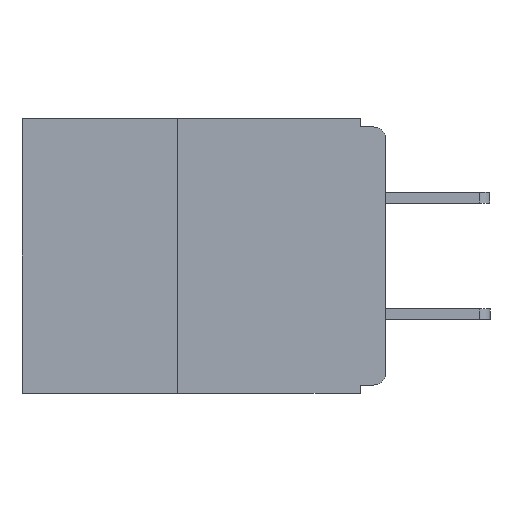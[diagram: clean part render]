
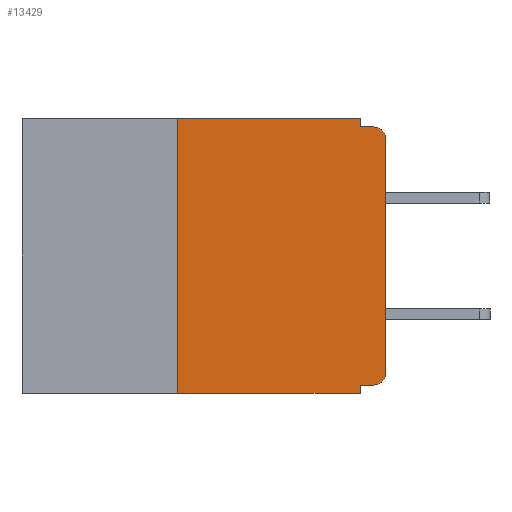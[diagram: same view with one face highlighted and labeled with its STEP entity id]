
A CAD part, left-side view. The second image highlights one B-rep face of the part: STEP entity #13429.
In plain terms, the highlighted planar face has unit normal (-1, 0, 0).
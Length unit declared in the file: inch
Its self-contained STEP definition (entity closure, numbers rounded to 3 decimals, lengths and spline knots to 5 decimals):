
#54 = CARTESIAN_POINT ( 'NONE',  ( 0., 0.437, -0.33 ) ) ;
#122 = DIRECTION ( 'NONE',  ( 0., -1., 0. ) ) ;
#486 = CIRCLE ( 'NONE', #9799, 0.015 ) ;
#499 = ORIENTED_EDGE ( 'NONE', *, *, #11029, .F. ) ;
#587 = CARTESIAN_POINT ( 'NONE',  ( 0., 0.015, -0.01 ) ) ;
#753 = VERTEX_POINT ( 'NONE', #5445 ) ;
#868 = VECTOR ( 'NONE', #995, 39.37008 ) ;
#995 = DIRECTION ( 'NONE',  ( 0., 0., 1. ) ) ;
#1781 = DIRECTION ( 'NONE',  ( 0., 0., -1. ) ) ;
#1915 = VERTEX_POINT ( 'NONE', #16449 ) ;
#2059 = CARTESIAN_POINT ( 'NONE',  ( 0., 0.25, 0. ) ) ;
#2167 = CARTESIAN_POINT ( 'NONE',  ( 0., 0.25, -0.33 ) ) ;
#2511 = EDGE_CURVE ( 'NONE', #12281, #8519, #7254, .T. ) ;
#2541 = DIRECTION ( 'NONE',  ( -1., 0., 0. ) ) ;
#2707 = ORIENTED_EDGE ( 'NONE', *, *, #2511, .F. ) ;
#3223 = EDGE_LOOP ( 'NONE', ( #7993, #9300, #13137, #499, #2707, #6318, #10395, #12358, #15244, #6492 ) ) ;
#3618 = VERTEX_POINT ( 'NONE', #2167 ) ;
#4325 = VERTEX_POINT ( 'NONE', #587 ) ;
#4345 = VERTEX_POINT ( 'NONE', #17056 ) ;
#4640 = PLANE ( 'NONE',  #17543 ) ;
#4710 = LINE ( 'NONE', #15210, #7951 ) ;
#4816 = CARTESIAN_POINT ( 'NONE',  ( 0., 0.015, -0.025 ) ) ;
#4822 = DIRECTION ( 'NONE',  ( 0., 0., 1. ) ) ;
#4953 = CIRCLE ( 'NONE', #10786, 0.015 ) ;
#5091 = CARTESIAN_POINT ( 'NONE',  ( 0., 0.031, -0.33 ) ) ;
#5439 = EDGE_CURVE ( 'NONE', #3618, #753, #10393, .T. ) ;
#5445 = CARTESIAN_POINT ( 'NONE',  ( 0., 0.031, -0.33 ) ) ;
#5471 = CARTESIAN_POINT ( 'NONE',  ( 0., 0.015, -0.32 ) ) ;
#5827 = LINE ( 'NONE', #7615, #11805 ) ;
#6002 = CARTESIAN_POINT ( 'NONE',  ( 0., 0.031, 0. ) ) ;
#6135 = DIRECTION ( 'NONE',  ( 0., 0., -1. ) ) ;
#6243 = DIRECTION ( 'NONE',  ( 0., 0., -1. ) ) ;
#6318 = ORIENTED_EDGE ( 'NONE', *, *, #15006, .F. ) ;
#6480 = VERTEX_POINT ( 'NONE', #5471 ) ;
#6492 = ORIENTED_EDGE ( 'NONE', *, *, #16210, .T. ) ;
#6711 = VECTOR ( 'NONE', #1781, 39.37008 ) ;
#7254 = LINE ( 'NONE', #11456, #10464 ) ;
#7615 = CARTESIAN_POINT ( 'NONE',  ( 0., 0., -0.32 ) ) ;
#7951 = VECTOR ( 'NONE', #8527, 39.37008 ) ;
#7993 = ORIENTED_EDGE ( 'NONE', *, *, #11112, .T. ) ;
#8242 = CARTESIAN_POINT ( 'NONE',  ( 0., 0.031, -0.01 ) ) ;
#8519 = VERTEX_POINT ( 'NONE', #16820 ) ;
#8527 = DIRECTION ( 'NONE',  ( 0., -1., 0. ) ) ;
#8535 = EDGE_CURVE ( 'NONE', #6480, #4345, #5827, .T. ) ;
#8560 = LINE ( 'NONE', #12920, #15266 ) ;
#8633 = EDGE_CURVE ( 'NONE', #4345, #753, #10525, .T. ) ;
#9122 = FACE_OUTER_BOUND ( 'NONE', #3223, .T. ) ;
#9300 = ORIENTED_EDGE ( 'NONE', *, *, #12245, .T. ) ;
#9526 = VERTEX_POINT ( 'NONE', #8242 ) ;
#9799 = AXIS2_PLACEMENT_3D ( 'NONE', #4816, #14290, #6243 ) ;
#9873 = LINE ( 'NONE', #6002, #6711 ) ;
#10223 = CARTESIAN_POINT ( 'NONE',  ( 0., 0., -0.025 ) ) ;
#10393 = LINE ( 'NONE', #54, #16984 ) ;
#10395 = ORIENTED_EDGE ( 'NONE', *, *, #5439, .T. ) ;
#10464 = VECTOR ( 'NONE', #11515, 39.37008 ) ;
#10525 = LINE ( 'NONE', #5091, #13648 ) ;
#10786 = AXIS2_PLACEMENT_3D ( 'NONE', #10820, #2541, #12174 ) ;
#10820 = CARTESIAN_POINT ( 'NONE',  ( 0., 0.015, -0.305 ) ) ;
#10925 = EDGE_CURVE ( 'NONE', #9526, #4325, #4710, .T. ) ;
#11029 = EDGE_CURVE ( 'NONE', #8519, #9526, #9873, .T. ) ;
#11112 = EDGE_CURVE ( 'NONE', #1915, #13448, #8560, .T. ) ;
#11456 = CARTESIAN_POINT ( 'NONE',  ( 0., 0.437, 0. ) ) ;
#11515 = DIRECTION ( 'NONE',  ( 0., -1., 0. ) ) ;
#11548 = CARTESIAN_POINT ( 'NONE',  ( 0., 0.437, 0. ) ) ;
#11805 = VECTOR ( 'NONE', #15621, 39.37008 ) ;
#11888 = LINE ( 'NONE', #17209, #868 ) ;
#12174 = DIRECTION ( 'NONE',  ( 0., 0., -1. ) ) ;
#12245 = EDGE_CURVE ( 'NONE', #13448, #4325, #486, .T. ) ;
#12281 = VERTEX_POINT ( 'NONE', #2059 ) ;
#12358 = ORIENTED_EDGE ( 'NONE', *, *, #8633, .F. ) ;
#12920 = CARTESIAN_POINT ( 'NONE',  ( 0., 0., 0. ) ) ;
#13137 = ORIENTED_EDGE ( 'NONE', *, *, #10925, .F. ) ;
#13429 = ADVANCED_FACE ( 'NONE', ( #9122 ), #4640, .F. ) ;
#13448 = VERTEX_POINT ( 'NONE', #10223 ) ;
#13648 = VECTOR ( 'NONE', #15860, 39.37008 ) ;
#14184 = DIRECTION ( 'NONE',  ( 1., 0., 0. ) ) ;
#14290 = DIRECTION ( 'NONE',  ( -1., 0., 0. ) ) ;
#15006 = EDGE_CURVE ( 'NONE', #3618, #12281, #11888, .T. ) ;
#15210 = CARTESIAN_POINT ( 'NONE',  ( 0., 0., -0.01 ) ) ;
#15244 = ORIENTED_EDGE ( 'NONE', *, *, #8535, .F. ) ;
#15266 = VECTOR ( 'NONE', #4822, 39.37008 ) ;
#15621 = DIRECTION ( 'NONE',  ( 0., 1., 0. ) ) ;
#15860 = DIRECTION ( 'NONE',  ( 0., 0., -1. ) ) ;
#16210 = EDGE_CURVE ( 'NONE', #6480, #1915, #4953, .T. ) ;
#16449 = CARTESIAN_POINT ( 'NONE',  ( 0., 0., -0.305 ) ) ;
#16820 = CARTESIAN_POINT ( 'NONE',  ( 0., 0.031, 0. ) ) ;
#16984 = VECTOR ( 'NONE', #122, 39.37008 ) ;
#17056 = CARTESIAN_POINT ( 'NONE',  ( 0., 0.031, -0.32 ) ) ;
#17209 = CARTESIAN_POINT ( 'NONE',  ( 0., 0.25, -0.33 ) ) ;
#17543 = AXIS2_PLACEMENT_3D ( 'NONE', #11548, #14184, #6135 ) ;
